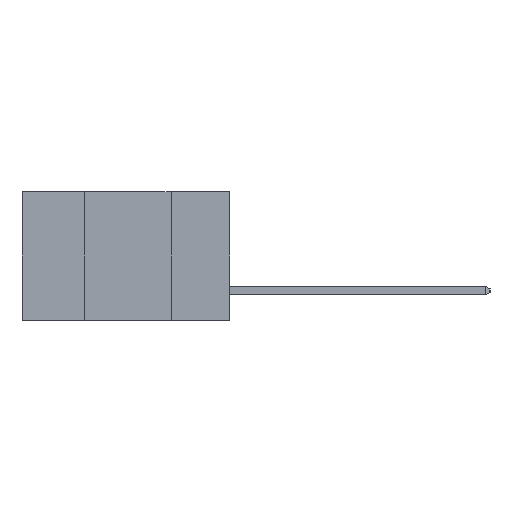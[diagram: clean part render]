
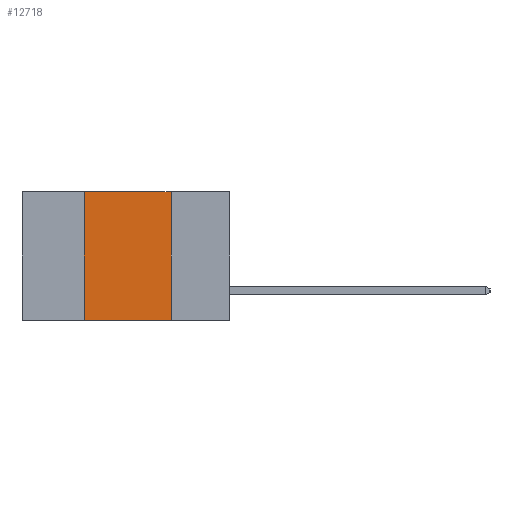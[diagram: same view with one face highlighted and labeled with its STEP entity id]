
A CAD part, left-side view. The second image highlights one B-rep face of the part: STEP entity #12718.
In plain terms, the highlighted planar face has unit normal (-1, 0, 0).
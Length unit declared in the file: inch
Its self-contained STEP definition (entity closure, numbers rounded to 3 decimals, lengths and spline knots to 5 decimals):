
#1616 = CARTESIAN_POINT ( 'NONE',  ( 0., 0.17, -0.37 ) ) ;
#1679 = ORIENTED_EDGE ( 'NONE', *, *, #14519, .T. ) ;
#2439 = ORIENTED_EDGE ( 'NONE', *, *, #20121, .F. ) ;
#3048 = LINE ( 'NONE', #20610, #20527 ) ;
#3186 = VECTOR ( 'NONE', #13343, 39.37008 ) ;
#3211 = DIRECTION ( 'NONE',  ( 0., -1., 0. ) ) ;
#4053 = ORIENTED_EDGE ( 'NONE', *, *, #18142, .F. ) ;
#4508 = CARTESIAN_POINT ( 'NONE',  ( 0., 0.42, -0.37 ) ) ;
#6029 = DIRECTION ( 'NONE',  ( 0., 0., -1. ) ) ;
#6512 = VERTEX_POINT ( 'NONE', #19091 ) ;
#6967 = AXIS2_PLACEMENT_3D ( 'NONE', #9513, #16693, #6029 ) ;
#7529 = VECTOR ( 'NONE', #18103, 39.37008 ) ;
#9513 = CARTESIAN_POINT ( 'NONE',  ( 0., 0.6, 0. ) ) ;
#9896 = VERTEX_POINT ( 'NONE', #4508 ) ;
#11491 = VECTOR ( 'NONE', #15976, 39.37008 ) ;
#12074 = LINE ( 'NONE', #14230, #11491 ) ;
#12718 = ADVANCED_FACE ( 'NONE', ( #16850 ), #14939, .F. ) ;
#13109 = LINE ( 'NONE', #16860, #3186 ) ;
#13343 = DIRECTION ( 'NONE',  ( 0., 0., -1. ) ) ;
#13394 = CARTESIAN_POINT ( 'NONE',  ( 0., 0.17, 0. ) ) ;
#14230 = CARTESIAN_POINT ( 'NONE',  ( 0., 0.6, -0.37 ) ) ;
#14519 = EDGE_CURVE ( 'NONE', #9896, #19387, #12074, .T. ) ;
#14710 = EDGE_CURVE ( 'NONE', #9896, #6512, #16477, .T. ) ;
#14777 = EDGE_LOOP ( 'NONE', ( #4053, #2439, #14860, #1679 ) ) ;
#14860 = ORIENTED_EDGE ( 'NONE', *, *, #14710, .F. ) ;
#14939 = PLANE ( 'NONE',  #6967 ) ;
#15976 = DIRECTION ( 'NONE',  ( 0., -1., 0. ) ) ;
#16477 = LINE ( 'NONE', #21562, #7529 ) ;
#16693 = DIRECTION ( 'NONE',  ( 1., 0., 0. ) ) ;
#16850 = FACE_OUTER_BOUND ( 'NONE', #14777, .T. ) ;
#16860 = CARTESIAN_POINT ( 'NONE',  ( 0., 0.17, 0. ) ) ;
#18103 = DIRECTION ( 'NONE',  ( 0., 0., 1. ) ) ;
#18142 = EDGE_CURVE ( 'NONE', #20025, #19387, #13109, .T. ) ;
#19091 = CARTESIAN_POINT ( 'NONE',  ( 0., 0.42, 0. ) ) ;
#19387 = VERTEX_POINT ( 'NONE', #1616 ) ;
#20025 = VERTEX_POINT ( 'NONE', #13394 ) ;
#20121 = EDGE_CURVE ( 'NONE', #6512, #20025, #3048, .T. ) ;
#20527 = VECTOR ( 'NONE', #3211, 39.37008 ) ;
#20610 = CARTESIAN_POINT ( 'NONE',  ( 0., 0.6, 0. ) ) ;
#21562 = CARTESIAN_POINT ( 'NONE',  ( 0., 0.42, 0. ) ) ;
